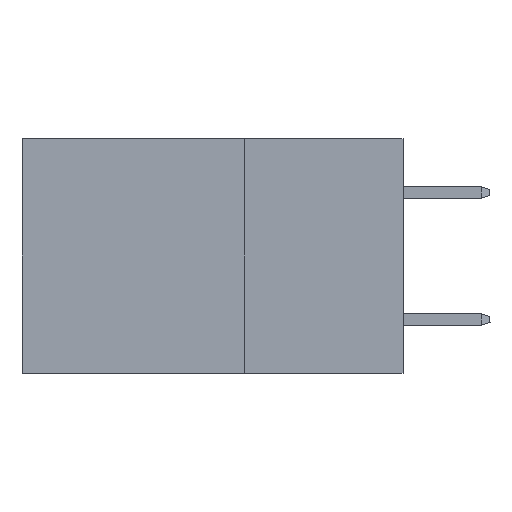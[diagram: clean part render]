
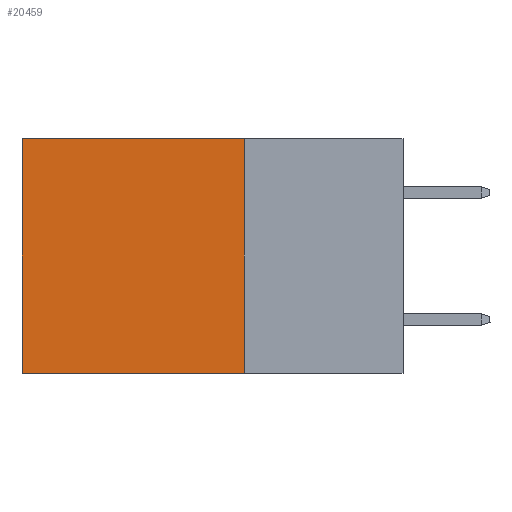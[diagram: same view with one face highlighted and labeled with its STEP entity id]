
A CAD part, left-side view. The second image highlights one B-rep face of the part: STEP entity #20459.
In plain terms, the highlighted planar face has unit normal (-1, 0, 0).
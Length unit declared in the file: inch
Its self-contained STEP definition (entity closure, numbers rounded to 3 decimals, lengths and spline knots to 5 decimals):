
#2256 = CARTESIAN_POINT ( 'NONE',  ( 0.2875, 0.25, 0. ) ) ;
#3256 = DIRECTION ( 'NONE',  ( 0., 1., 0. ) ) ;
#5828 = ORIENTED_EDGE ( 'NONE', *, *, #22494, .F. ) ;
#7290 = DIRECTION ( 'NONE',  ( 1., 0., 0. ) ) ;
#7428 = VECTOR ( 'NONE', #19747, 39.37008 ) ;
#7758 = EDGE_CURVE ( 'NONE', #16147, #20563, #8644, .T. ) ;
#8644 = LINE ( 'NONE', #13821, #17363 ) ;
#10742 = CARTESIAN_POINT ( 'NONE',  ( 0.2875, 0.6, -0.37 ) ) ;
#11242 = VECTOR ( 'NONE', #20550, 39.37008 ) ;
#13821 = CARTESIAN_POINT ( 'NONE',  ( 0.2875, 0.25, 0. ) ) ;
#13889 = CARTESIAN_POINT ( 'NONE',  ( 0.2875, 0.25, -0.37 ) ) ;
#14810 = EDGE_CURVE ( 'NONE', #16147, #27408, #30274, .T. ) ;
#15047 = CARTESIAN_POINT ( 'NONE',  ( 0.2875, 0.6, 0. ) ) ;
#16147 = VERTEX_POINT ( 'NONE', #29921 ) ;
#16230 = EDGE_CURVE ( 'NONE', #27408, #30950, #25729, .T. ) ;
#17363 = VECTOR ( 'NONE', #26342, 39.37008 ) ;
#18860 = ORIENTED_EDGE ( 'NONE', *, *, #14810, .T. ) ;
#19747 = DIRECTION ( 'NONE',  ( 0., 1., 0. ) ) ;
#20295 = CARTESIAN_POINT ( 'NONE',  ( 0.2875, 0.25, -0.37 ) ) ;
#20342 = ORIENTED_EDGE ( 'NONE', *, *, #7758, .F. ) ;
#20459 = ADVANCED_FACE ( 'NONE', ( #22141 ), #30159, .F. ) ;
#20550 = DIRECTION ( 'NONE',  ( 0., 0., -1. ) ) ;
#20563 = VERTEX_POINT ( 'NONE', #20295 ) ;
#20940 = AXIS2_PLACEMENT_3D ( 'NONE', #32342, #7290, #29832 ) ;
#21520 = ORIENTED_EDGE ( 'NONE', *, *, #16230, .T. ) ;
#21574 = LINE ( 'NONE', #13889, #23175 ) ;
#21990 = CARTESIAN_POINT ( 'NONE',  ( 0.2875, 0.6, 0. ) ) ;
#22141 = FACE_OUTER_BOUND ( 'NONE', #23378, .T. ) ;
#22494 = EDGE_CURVE ( 'NONE', #20563, #30950, #21574, .T. ) ;
#23175 = VECTOR ( 'NONE', #3256, 39.37008 ) ;
#23378 = EDGE_LOOP ( 'NONE', ( #21520, #5828, #20342, #18860 ) ) ;
#25729 = LINE ( 'NONE', #15047, #11242 ) ;
#26342 = DIRECTION ( 'NONE',  ( 0., 0., -1. ) ) ;
#27408 = VERTEX_POINT ( 'NONE', #21990 ) ;
#29832 = DIRECTION ( 'NONE',  ( 0., 0., -1. ) ) ;
#29921 = CARTESIAN_POINT ( 'NONE',  ( 0.2875, 0.25, 0. ) ) ;
#30159 = PLANE ( 'NONE',  #20940 ) ;
#30274 = LINE ( 'NONE', #2256, #7428 ) ;
#30950 = VERTEX_POINT ( 'NONE', #10742 ) ;
#32342 = CARTESIAN_POINT ( 'NONE',  ( 0.2875, 0.25, 0. ) ) ;
